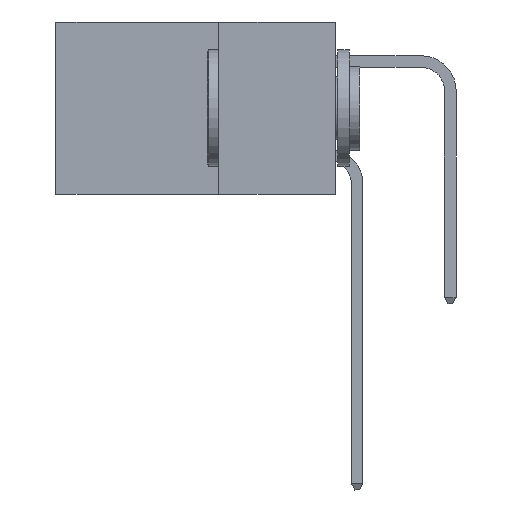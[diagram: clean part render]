
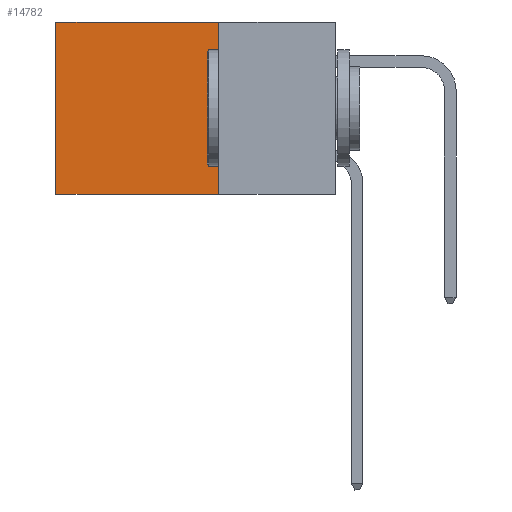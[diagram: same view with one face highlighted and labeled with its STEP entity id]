
A CAD part, left-side view. The second image highlights one B-rep face of the part: STEP entity #14782.
In plain terms, the highlighted planar face has unit normal (-1, 0, 0).
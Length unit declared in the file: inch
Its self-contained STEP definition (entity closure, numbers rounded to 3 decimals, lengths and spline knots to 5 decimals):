
#849 = DIRECTION ( 'NONE',  ( 0., 0., -1. ) ) ;
#2058 = LINE ( 'NONE', #33947, #10333 ) ;
#2591 = LINE ( 'NONE', #17967, #27478 ) ;
#2972 = CARTESIAN_POINT ( 'NONE',  ( 0.2875, 0.25, -0.37 ) ) ;
#3592 = DIRECTION ( 'NONE',  ( 0., 1., 0. ) ) ;
#4867 = CARTESIAN_POINT ( 'NONE',  ( 0.2875, 0.25, 0. ) ) ;
#6470 = ORIENTED_EDGE ( 'NONE', *, *, #38564, .F. ) ;
#6826 = VECTOR ( 'NONE', #3592, 39.37008 ) ;
#6998 = EDGE_CURVE ( 'NONE', #11214, #40409, #39638, .T. ) ;
#7660 = EDGE_CURVE ( 'NONE', #39246, #14421, #29110, .T. ) ;
#8023 = PLANE ( 'NONE',  #21722 ) ;
#10192 = CARTESIAN_POINT ( 'NONE',  ( 0.2875, 0.6, -0.37 ) ) ;
#10333 = VECTOR ( 'NONE', #849, 39.37008 ) ;
#10713 = CARTESIAN_POINT ( 'NONE',  ( 0.2875, 0.25, 0. ) ) ;
#11214 = VERTEX_POINT ( 'NONE', #2972 ) ;
#11610 = ORIENTED_EDGE ( 'NONE', *, *, #7660, .T. ) ;
#14421 = VERTEX_POINT ( 'NONE', #20452 ) ;
#14782 = ADVANCED_FACE ( 'NONE', ( #20833 ), #8023, .F. ) ;
#16016 = EDGE_CURVE ( 'NONE', #14421, #40409, #2058, .T. ) ;
#17967 = CARTESIAN_POINT ( 'NONE',  ( 0.2875, 0.25, 0. ) ) ;
#20367 = CARTESIAN_POINT ( 'NONE',  ( 0.2875, 0.25, -0.37 ) ) ;
#20452 = CARTESIAN_POINT ( 'NONE',  ( 0.2875, 0.6, 0. ) ) ;
#20833 = FACE_OUTER_BOUND ( 'NONE', #21282, .T. ) ;
#21282 = EDGE_LOOP ( 'NONE', ( #35037, #29981, #6470, #11610 ) ) ;
#21722 = AXIS2_PLACEMENT_3D ( 'NONE', #4867, #31731, #34623 ) ;
#23393 = DIRECTION ( 'NONE',  ( 0., 1., 0. ) ) ;
#27478 = VECTOR ( 'NONE', #28150, 39.37008 ) ;
#28150 = DIRECTION ( 'NONE',  ( 0., 0., -1. ) ) ;
#29110 = LINE ( 'NONE', #40018, #34361 ) ;
#29981 = ORIENTED_EDGE ( 'NONE', *, *, #6998, .F. ) ;
#31731 = DIRECTION ( 'NONE',  ( 1., 0., 0. ) ) ;
#33947 = CARTESIAN_POINT ( 'NONE',  ( 0.2875, 0.6, 0. ) ) ;
#34361 = VECTOR ( 'NONE', #23393, 39.37008 ) ;
#34623 = DIRECTION ( 'NONE',  ( 0., 0., -1. ) ) ;
#35037 = ORIENTED_EDGE ( 'NONE', *, *, #16016, .T. ) ;
#38564 = EDGE_CURVE ( 'NONE', #39246, #11214, #2591, .T. ) ;
#39246 = VERTEX_POINT ( 'NONE', #10713 ) ;
#39638 = LINE ( 'NONE', #20367, #6826 ) ;
#40018 = CARTESIAN_POINT ( 'NONE',  ( 0.2875, 0.25, 0. ) ) ;
#40409 = VERTEX_POINT ( 'NONE', #10192 ) ;
